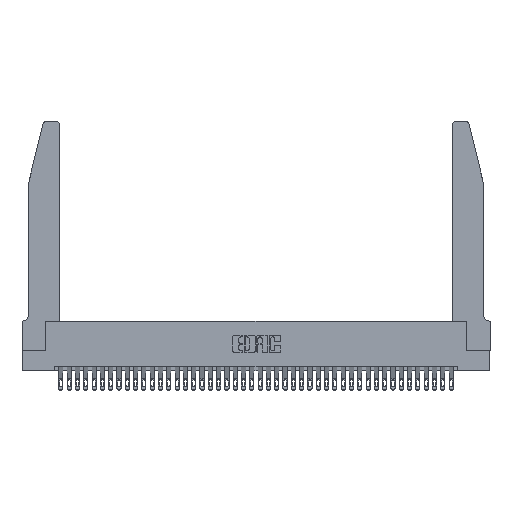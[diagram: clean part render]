
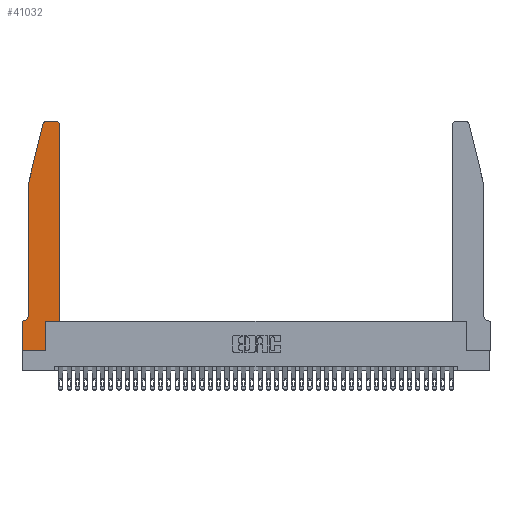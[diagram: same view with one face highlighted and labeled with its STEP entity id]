
A CAD part, top view. The second image highlights one B-rep face of the part: STEP entity #41032.
In plain terms, the highlighted planar face has unit normal (0, 0, 1).
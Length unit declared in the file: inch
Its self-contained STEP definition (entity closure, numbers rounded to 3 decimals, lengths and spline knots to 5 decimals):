
#64 = DIRECTION ( 'NONE',  ( 1., 0., 0. ) ) ;
#509 = VECTOR ( 'NONE', #21721, 39.37008 ) ;
#924 = CARTESIAN_POINT ( 'NONE',  ( 0.2605, 2.75, 0.37 ) ) ;
#1320 = VERTEX_POINT ( 'NONE', #16803 ) ;
#1562 = DIRECTION ( 'NONE',  ( 0., 0., 1. ) ) ;
#2683 = CARTESIAN_POINT ( 'NONE',  ( 0.2865, 0.35, 0.37 ) ) ;
#2887 = CARTESIAN_POINT ( 'NONE',  ( 0.0755, 2., 0.37 ) ) ;
#2982 = EDGE_CURVE ( 'NONE', #33515, #17234, #5520, .T. ) ;
#3276 = VECTOR ( 'NONE', #20034, 39.37008 ) ;
#3897 = ORIENTED_EDGE ( 'NONE', *, *, #10197, .T. ) ;
#5262 = CARTESIAN_POINT ( 'NONE',  ( 0.284, 2.75, 0.37 ) ) ;
#5520 = LINE ( 'NONE', #2887, #8099 ) ;
#5642 = CARTESIAN_POINT ( 'NONE',  ( 0.0055, 0.35, 0.37 ) ) ;
#6112 = EDGE_CURVE ( 'NONE', #38270, #17220, #9875, .T. ) ;
#6675 = VECTOR ( 'NONE', #15864, 39.37008 ) ;
#6917 = ORIENTED_EDGE ( 'NONE', *, *, #13968, .T. ) ;
#7834 = CARTESIAN_POINT ( 'NONE',  ( 0., 0.35, 0.37 ) ) ;
#8099 = VECTOR ( 'NONE', #38287, 39.37008 ) ;
#8231 = VERTEX_POINT ( 'NONE', #30009 ) ;
#8703 = LINE ( 'NONE', #28473, #6675 ) ;
#9085 = VERTEX_POINT ( 'NONE', #2683 ) ;
#9875 = LINE ( 'NONE', #14722, #34647 ) ;
#9965 = ORIENTED_EDGE ( 'NONE', *, *, #21336, .T. ) ;
#10197 = EDGE_CURVE ( 'NONE', #17234, #15036, #28132, .T. ) ;
#10218 = CARTESIAN_POINT ( 'NONE',  ( 0.284, 2.72, 0.37 ) ) ;
#10819 = EDGE_CURVE ( 'NONE', #23240, #13535, #34636, .T. ) ;
#10942 = FACE_OUTER_BOUND ( 'NONE', #16371, .T. ) ;
#11143 = CARTESIAN_POINT ( 'NONE',  ( 0.25487, 2.72718, 0.37 ) ) ;
#12213 = LINE ( 'NONE', #25965, #26873 ) ;
#12873 = CARTESIAN_POINT ( 'NONE',  ( 0.4505, 2.72, 0.37 ) ) ;
#12918 = DIRECTION ( 'NONE',  ( 0., 0., 1. ) ) ;
#13535 = VERTEX_POINT ( 'NONE', #11143 ) ;
#13696 = VECTOR ( 'NONE', #26724, 39.37008 ) ;
#13968 = EDGE_CURVE ( 'NONE', #1320, #19721, #40951, .T. ) ;
#14195 = DIRECTION ( 'NONE',  ( 0., 0., -1. ) ) ;
#14722 = CARTESIAN_POINT ( 'NONE',  ( 0.4505, 0.35, 0.37 ) ) ;
#15036 = VERTEX_POINT ( 'NONE', #5642 ) ;
#15864 = DIRECTION ( 'NONE',  ( 0., 1., 0. ) ) ;
#15958 = LINE ( 'NONE', #924, #3276 ) ;
#16205 = DIRECTION ( 'NONE',  ( 1., 0., 0. ) ) ;
#16371 = EDGE_LOOP ( 'NONE', ( #25188, #36921, #38341, #39169, #3897, #28237, #36201, #6917, #20250, #39122, #22818, #9965 ) ) ;
#16803 = CARTESIAN_POINT ( 'NONE',  ( 0., 0., 0.37 ) ) ;
#17220 = VERTEX_POINT ( 'NONE', #12873 ) ;
#17234 = VERTEX_POINT ( 'NONE', #28895 ) ;
#18001 = EDGE_CURVE ( 'NONE', #13535, #33515, #38041, .T. ) ;
#18316 = EDGE_CURVE ( 'NONE', #15036, #18753, #34971, .T. ) ;
#18753 = VERTEX_POINT ( 'NONE', #7834 ) ;
#19721 = VERTEX_POINT ( 'NONE', #25845 ) ;
#20034 = DIRECTION ( 'NONE',  ( -1., 0., 0. ) ) ;
#20250 = ORIENTED_EDGE ( 'NONE', *, *, #32973, .T. ) ;
#20398 = EDGE_CURVE ( 'NONE', #18753, #1320, #31437, .T. ) ;
#20646 = VECTOR ( 'NONE', #16205, 39.37008 ) ;
#21336 = EDGE_CURVE ( 'NONE', #17220, #8231, #22759, .T. ) ;
#21414 = CARTESIAN_POINT ( 'NONE',  ( 0.4505, 0.35, 0.37 ) ) ;
#21721 = DIRECTION ( 'NONE',  ( -1., 0., 0. ) ) ;
#22759 = CIRCLE ( 'NONE', #36915, 0.03 ) ;
#22818 = ORIENTED_EDGE ( 'NONE', *, *, #6112, .T. ) ;
#23240 = VERTEX_POINT ( 'NONE', #5262 ) ;
#24067 = DIRECTION ( 'NONE',  ( 1., 0., 0. ) ) ;
#24353 = PLANE ( 'NONE',  #25475 ) ;
#24595 = CARTESIAN_POINT ( 'NONE',  ( 0.0755, 2., 0.37 ) ) ;
#24882 = VECTOR ( 'NONE', #35719, 39.37008 ) ;
#24980 = DIRECTION ( 'NONE',  ( 0., 0., 1. ) ) ;
#25188 = ORIENTED_EDGE ( 'NONE', *, *, #30735, .T. ) ;
#25475 = AXIS2_PLACEMENT_3D ( 'NONE', #33940, #1562, #24067 ) ;
#25845 = CARTESIAN_POINT ( 'NONE',  ( 0.2865, 0., 0.37 ) ) ;
#25935 = EDGE_CURVE ( 'NONE', #9085, #38270, #12213, .T. ) ;
#25965 = CARTESIAN_POINT ( 'NONE',  ( 0.4505, 0.35, 0.37 ) ) ;
#26724 = DIRECTION ( 'NONE',  ( 0., -1., 0. ) ) ;
#26873 = VECTOR ( 'NONE', #64, 39.37008 ) ;
#28132 = CIRCLE ( 'NONE', #35419, 0.07 ) ;
#28237 = ORIENTED_EDGE ( 'NONE', *, *, #18316, .T. ) ;
#28473 = CARTESIAN_POINT ( 'NONE',  ( 0.2865, 0.35, 0.37 ) ) ;
#28799 = DIRECTION ( 'NONE',  ( 1., 0., 0. ) ) ;
#28895 = CARTESIAN_POINT ( 'NONE',  ( 0.0755, 0.42, 0.37 ) ) ;
#30009 = CARTESIAN_POINT ( 'NONE',  ( 0.4205, 2.75, 0.37 ) ) ;
#30735 = EDGE_CURVE ( 'NONE', #8231, #23240, #15958, .T. ) ;
#31437 = LINE ( 'NONE', #40189, #13696 ) ;
#32480 = CARTESIAN_POINT ( 'NONE',  ( 0.0755, 2., 0.37 ) ) ;
#32829 = DIRECTION ( 'NONE',  ( 1., 0., 0. ) ) ;
#32973 = EDGE_CURVE ( 'NONE', #19721, #9085, #8703, .T. ) ;
#33515 = VERTEX_POINT ( 'NONE', #24595 ) ;
#33540 = CARTESIAN_POINT ( 'NONE',  ( 0.0055, 0.42, 0.37 ) ) ;
#33940 = CARTESIAN_POINT ( 'NONE',  ( 0., 0.35, 0.37 ) ) ;
#34636 = CIRCLE ( 'NONE', #39529, 0.03 ) ;
#34647 = VECTOR ( 'NONE', #37319, 39.37008 ) ;
#34971 = LINE ( 'NONE', #41136, #509 ) ;
#35144 = CARTESIAN_POINT ( 'NONE',  ( 0., 0., 0.37 ) ) ;
#35419 = AXIS2_PLACEMENT_3D ( 'NONE', #33540, #14195, #37093 ) ;
#35719 = DIRECTION ( 'NONE',  ( -0.239, -0.971, 0. ) ) ;
#36201 = ORIENTED_EDGE ( 'NONE', *, *, #20398, .T. ) ;
#36915 = AXIS2_PLACEMENT_3D ( 'NONE', #41682, #24980, #28799 ) ;
#36921 = ORIENTED_EDGE ( 'NONE', *, *, #10819, .T. ) ;
#37093 = DIRECTION ( 'NONE',  ( -1., 0., 0. ) ) ;
#37319 = DIRECTION ( 'NONE',  ( 0., 1., 0. ) ) ;
#38041 = LINE ( 'NONE', #32480, #24882 ) ;
#38270 = VERTEX_POINT ( 'NONE', #21414 ) ;
#38287 = DIRECTION ( 'NONE',  ( 0., -1., 0. ) ) ;
#38341 = ORIENTED_EDGE ( 'NONE', *, *, #18001, .T. ) ;
#39122 = ORIENTED_EDGE ( 'NONE', *, *, #25935, .T. ) ;
#39169 = ORIENTED_EDGE ( 'NONE', *, *, #2982, .T. ) ;
#39529 = AXIS2_PLACEMENT_3D ( 'NONE', #10218, #12918, #32829 ) ;
#40189 = CARTESIAN_POINT ( 'NONE',  ( 0., 0., 0.37 ) ) ;
#40951 = LINE ( 'NONE', #35144, #20646 ) ;
#41032 = ADVANCED_FACE ( 'NONE', ( #10942 ), #24353, .T. ) ;
#41136 = CARTESIAN_POINT ( 'NONE',  ( 0.0755, 0.35, 0.37 ) ) ;
#41682 = CARTESIAN_POINT ( 'NONE',  ( 0.4205, 2.72, 0.37 ) ) ;
